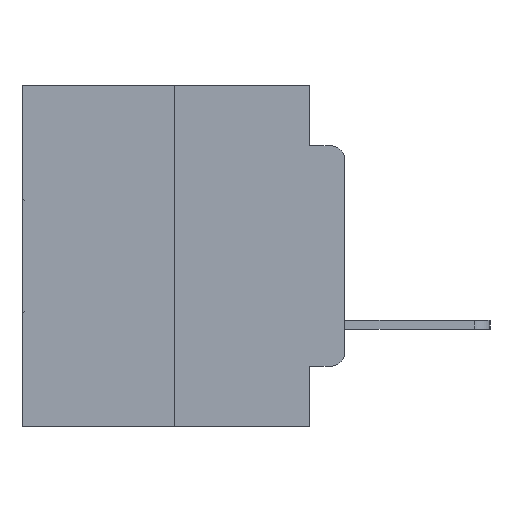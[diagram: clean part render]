
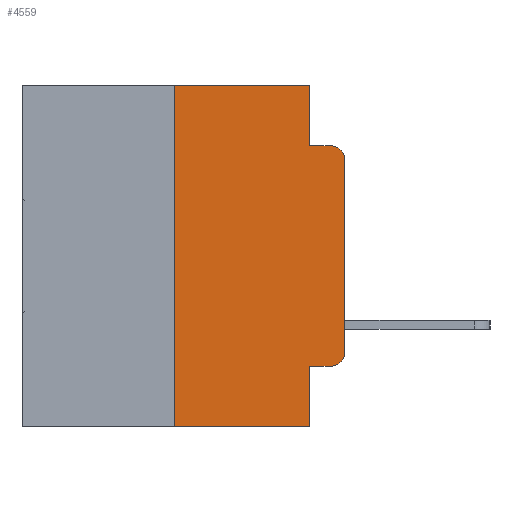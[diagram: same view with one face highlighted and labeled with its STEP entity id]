
A CAD part, left-side view. The second image highlights one B-rep face of the part: STEP entity #4559.
In plain terms, the highlighted planar face has unit normal (-1, 0, 0).
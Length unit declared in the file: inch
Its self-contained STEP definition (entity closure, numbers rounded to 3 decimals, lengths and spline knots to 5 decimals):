
#569 = DIRECTION ( 'NONE',  ( 0., -1., 0. ) ) ;
#589 = VECTOR ( 'NONE', #10679, 39.37008 ) ;
#595 = CARTESIAN_POINT ( 'NONE',  ( 0., 0.02, -0.4115 ) ) ;
#959 = LINE ( 'NONE', #16355, #7853 ) ;
#1706 = EDGE_CURVE ( 'NONE', #22138, #19788, #26365, .T. ) ;
#2559 = ORIENTED_EDGE ( 'NONE', *, *, #4523, .T. ) ;
#3010 = ORIENTED_EDGE ( 'NONE', *, *, #27853, .T. ) ;
#3259 = VERTEX_POINT ( 'NONE', #20245 ) ;
#3836 = DIRECTION ( 'NONE',  ( 0., 0., 1. ) ) ;
#4523 = EDGE_CURVE ( 'NONE', #17552, #8967, #22123, .T. ) ;
#4559 = ADVANCED_FACE ( 'NONE', ( #10612 ), #17372, .F. ) ;
#4655 = VECTOR ( 'NONE', #17940, 39.37008 ) ;
#4662 = ORIENTED_EDGE ( 'NONE', *, *, #12222, .F. ) ;
#4668 = CARTESIAN_POINT ( 'NONE',  ( 0., 0.051, 0. ) ) ;
#4697 = CIRCLE ( 'NONE', #25902, 0.02 ) ;
#6118 = LINE ( 'NONE', #25780, #589 ) ;
#6511 = CARTESIAN_POINT ( 'NONE',  ( 0., 0.051, -0.5 ) ) ;
#6957 = LINE ( 'NONE', #17200, #12242 ) ;
#6996 = EDGE_CURVE ( 'NONE', #26802, #22138, #6957, .T. ) ;
#7607 = CARTESIAN_POINT ( 'NONE',  ( 0., 0.051, -0.4115 ) ) ;
#7853 = VECTOR ( 'NONE', #569, 39.37008 ) ;
#8250 = AXIS2_PLACEMENT_3D ( 'NONE', #11685, #25664, #25636 ) ;
#8967 = VERTEX_POINT ( 'NONE', #6511 ) ;
#9894 = LINE ( 'NONE', #23265, #20786 ) ;
#10244 = DIRECTION ( 'NONE',  ( 0., 0., 1. ) ) ;
#10294 = ORIENTED_EDGE ( 'NONE', *, *, #23036, .T. ) ;
#10612 = FACE_OUTER_BOUND ( 'NONE', #25490, .T. ) ;
#10679 = DIRECTION ( 'NONE',  ( 0., -1., 0. ) ) ;
#11022 = ORIENTED_EDGE ( 'NONE', *, *, #13157, .F. ) ;
#11650 = VECTOR ( 'NONE', #27128, 39.37008 ) ;
#11685 = CARTESIAN_POINT ( 'NONE',  ( 0., 0.02, -0.1085 ) ) ;
#12222 = EDGE_CURVE ( 'NONE', #27554, #3259, #16498, .T. ) ;
#12242 = VECTOR ( 'NONE', #3836, 39.37008 ) ;
#12564 = DIRECTION ( 'NONE',  ( -1., 0., 0. ) ) ;
#12608 = EDGE_CURVE ( 'NONE', #3259, #19788, #6118, .T. ) ;
#12835 = CARTESIAN_POINT ( 'NONE',  ( 0., 0.051, 0. ) ) ;
#12923 = DIRECTION ( 'NONE',  ( 0., 0., -1. ) ) ;
#13072 = VERTEX_POINT ( 'NONE', #18696 ) ;
#13157 = EDGE_CURVE ( 'NONE', #17552, #27684, #9894, .T. ) ;
#13575 = DIRECTION ( 'NONE',  ( 0., -1., 0. ) ) ;
#13603 = CARTESIAN_POINT ( 'NONE',  ( 0., 0.473, -0.5 ) ) ;
#13701 = CARTESIAN_POINT ( 'NONE',  ( 0., 0.051, 0. ) ) ;
#14583 = DIRECTION ( 'NONE',  ( 1., 0., 0. ) ) ;
#14605 = DIRECTION ( 'NONE',  ( 0., 0., -1. ) ) ;
#14828 = CARTESIAN_POINT ( 'NONE',  ( 0., 0., -0.1085 ) ) ;
#15963 = ORIENTED_EDGE ( 'NONE', *, *, #19591, .F. ) ;
#15968 = EDGE_CURVE ( 'NONE', #27684, #27554, #959, .T. ) ;
#16207 = CARTESIAN_POINT ( 'NONE',  ( 0., 0.473, 0. ) ) ;
#16255 = CARTESIAN_POINT ( 'NONE',  ( 0., 0.25, 0. ) ) ;
#16330 = CARTESIAN_POINT ( 'NONE',  ( 0., 0.25, -0.5 ) ) ;
#16355 = CARTESIAN_POINT ( 'NONE',  ( 0., 0.473, 0. ) ) ;
#16429 = VECTOR ( 'NONE', #13575, 39.37008 ) ;
#16498 = LINE ( 'NONE', #13701, #4655 ) ;
#17200 = CARTESIAN_POINT ( 'NONE',  ( 0., 0., 0. ) ) ;
#17372 = PLANE ( 'NONE',  #19827 ) ;
#17449 = CARTESIAN_POINT ( 'NONE',  ( 0., 0., -0.3915 ) ) ;
#17552 = VERTEX_POINT ( 'NONE', #16330 ) ;
#17661 = VECTOR ( 'NONE', #12923, 39.37008 ) ;
#17940 = DIRECTION ( 'NONE',  ( 0., 0., -1. ) ) ;
#18696 = CARTESIAN_POINT ( 'NONE',  ( 0., 0.051, -0.4115 ) ) ;
#19591 = EDGE_CURVE ( 'NONE', #13072, #8967, #27626, .T. ) ;
#19788 = VERTEX_POINT ( 'NONE', #19943 ) ;
#19827 = AXIS2_PLACEMENT_3D ( 'NONE', #16207, #14583, #14605 ) ;
#19943 = CARTESIAN_POINT ( 'NONE',  ( 0., 0.02, -0.0885 ) ) ;
#20245 = CARTESIAN_POINT ( 'NONE',  ( 0., 0.051, -0.0885 ) ) ;
#20785 = VERTEX_POINT ( 'NONE', #595 ) ;
#20786 = VECTOR ( 'NONE', #10244, 39.37008 ) ;
#21943 = ORIENTED_EDGE ( 'NONE', *, *, #15968, .F. ) ;
#22123 = LINE ( 'NONE', #13603, #16429 ) ;
#22138 = VERTEX_POINT ( 'NONE', #14828 ) ;
#22549 = ORIENTED_EDGE ( 'NONE', *, *, #12608, .F. ) ;
#23036 = EDGE_CURVE ( 'NONE', #13072, #20785, #23837, .T. ) ;
#23265 = CARTESIAN_POINT ( 'NONE',  ( 0., 0.25, 0. ) ) ;
#23837 = LINE ( 'NONE', #7607, #11650 ) ;
#24275 = ORIENTED_EDGE ( 'NONE', *, *, #1706, .T. ) ;
#25429 = CARTESIAN_POINT ( 'NONE',  ( 0., 0.02, -0.3915 ) ) ;
#25490 = EDGE_LOOP ( 'NONE', ( #27593, #24275, #22549, #4662, #21943, #11022, #2559, #15963, #10294, #3010 ) ) ;
#25636 = DIRECTION ( 'NONE',  ( 0., 0., -1. ) ) ;
#25664 = DIRECTION ( 'NONE',  ( -1., 0., 0. ) ) ;
#25780 = CARTESIAN_POINT ( 'NONE',  ( 0., 0.051, -0.0885 ) ) ;
#25902 = AXIS2_PLACEMENT_3D ( 'NONE', #25429, #12564, #27508 ) ;
#26365 = CIRCLE ( 'NONE', #8250, 0.02 ) ;
#26802 = VERTEX_POINT ( 'NONE', #17449 ) ;
#27128 = DIRECTION ( 'NONE',  ( 0., -1., 0. ) ) ;
#27508 = DIRECTION ( 'NONE',  ( 0., 0., -1. ) ) ;
#27554 = VERTEX_POINT ( 'NONE', #4668 ) ;
#27593 = ORIENTED_EDGE ( 'NONE', *, *, #6996, .T. ) ;
#27626 = LINE ( 'NONE', #12835, #17661 ) ;
#27684 = VERTEX_POINT ( 'NONE', #16255 ) ;
#27853 = EDGE_CURVE ( 'NONE', #20785, #26802, #4697, .T. ) ;
